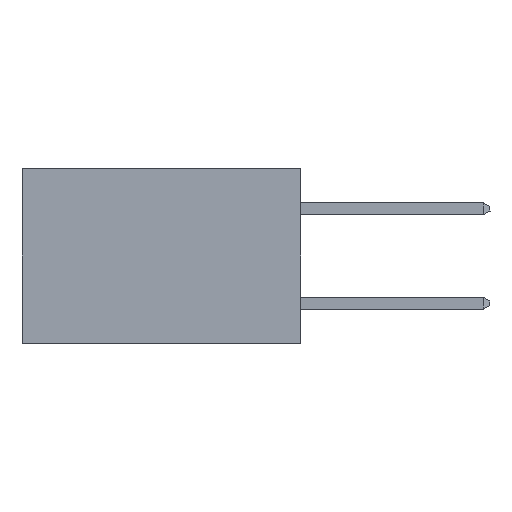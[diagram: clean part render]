
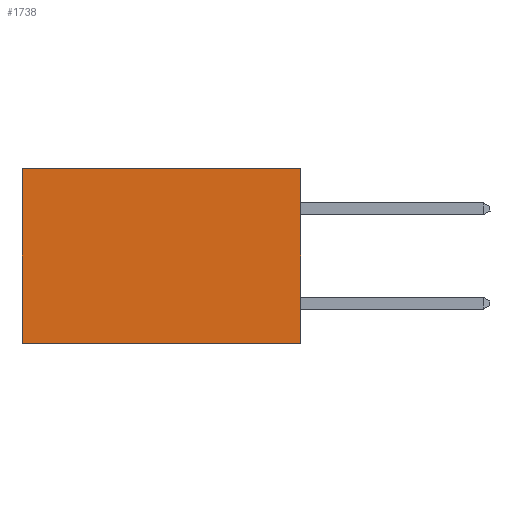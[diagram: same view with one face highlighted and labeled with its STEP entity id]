
A CAD part, left-side view. The second image highlights one B-rep face of the part: STEP entity #1738.
In plain terms, the highlighted planar face has unit normal (-1, 0, 0).
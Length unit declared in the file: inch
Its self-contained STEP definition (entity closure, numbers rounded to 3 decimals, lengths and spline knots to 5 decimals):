
#352 = EDGE_LOOP ( 'NONE', ( #1341, #3670, #1621, #6184 ) ) ;
#703 = VECTOR ( 'NONE', #1123, 39.37008 ) ;
#991 = EDGE_CURVE ( 'NONE', #9453, #3543, #2793, .T. ) ;
#1123 = DIRECTION ( 'NONE',  ( 0., 0., -1. ) ) ;
#1258 = EDGE_CURVE ( 'NONE', #4290, #8394, #7147, .T. ) ;
#1341 = ORIENTED_EDGE ( 'NONE', *, *, #1258, .T. ) ;
#1621 = ORIENTED_EDGE ( 'NONE', *, *, #991, .F. ) ;
#1738 = ADVANCED_FACE ( 'NONE', ( #2078 ), #8475, .F. ) ;
#1955 = DIRECTION ( 'NONE',  ( 0., 0., -1. ) ) ;
#2078 = FACE_OUTER_BOUND ( 'NONE', #352, .T. ) ;
#2099 = CARTESIAN_POINT ( 'NONE',  ( 0.277, 0.59, -0.37 ) ) ;
#2758 = CARTESIAN_POINT ( 'NONE',  ( 0.277, 0., -0.37 ) ) ;
#2793 = LINE ( 'NONE', #2758, #703 ) ;
#3080 = CARTESIAN_POINT ( 'NONE',  ( 0.277, 0.59, -0.37 ) ) ;
#3543 = VERTEX_POINT ( 'NONE', #7987 ) ;
#3670 = ORIENTED_EDGE ( 'NONE', *, *, #9620, .F. ) ;
#4290 = VERTEX_POINT ( 'NONE', #7500 ) ;
#5313 = LINE ( 'NONE', #6893, #7267 ) ;
#5946 = VECTOR ( 'NONE', #10523, 39.37008 ) ;
#6184 = ORIENTED_EDGE ( 'NONE', *, *, #8971, .T. ) ;
#6205 = LINE ( 'NONE', #6672, #5946 ) ;
#6672 = CARTESIAN_POINT ( 'NONE',  ( 0.277, 0., -0.37 ) ) ;
#6831 = DIRECTION ( 'NONE',  ( 0., 1., 0. ) ) ;
#6888 = VECTOR ( 'NONE', #1955, 39.37008 ) ;
#6893 = CARTESIAN_POINT ( 'NONE',  ( 0.277, 0., 0. ) ) ;
#7147 = LINE ( 'NONE', #3080, #6888 ) ;
#7267 = VECTOR ( 'NONE', #6831, 39.37008 ) ;
#7500 = CARTESIAN_POINT ( 'NONE',  ( 0.277, 0.59, 0. ) ) ;
#7909 = DIRECTION ( 'NONE',  ( 1., 0., 0. ) ) ;
#7925 = CARTESIAN_POINT ( 'NONE',  ( 0.277, 0., -0.37 ) ) ;
#7987 = CARTESIAN_POINT ( 'NONE',  ( 0.277, 0., -0.37 ) ) ;
#8394 = VERTEX_POINT ( 'NONE', #2099 ) ;
#8475 = PLANE ( 'NONE',  #10158 ) ;
#8971 = EDGE_CURVE ( 'NONE', #9453, #4290, #5313, .T. ) ;
#9453 = VERTEX_POINT ( 'NONE', #9639 ) ;
#9620 = EDGE_CURVE ( 'NONE', #3543, #8394, #6205, .T. ) ;
#9639 = CARTESIAN_POINT ( 'NONE',  ( 0.277, 0., 0. ) ) ;
#10158 = AXIS2_PLACEMENT_3D ( 'NONE', #7925, #7909, #10350 ) ;
#10350 = DIRECTION ( 'NONE',  ( 0., 0., -1. ) ) ;
#10523 = DIRECTION ( 'NONE',  ( 0., 1., 0. ) ) ;
